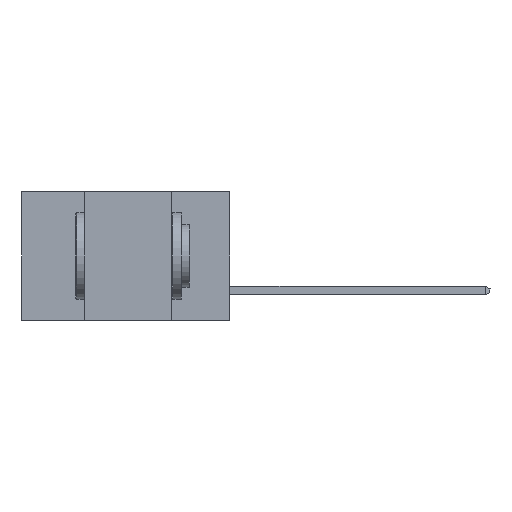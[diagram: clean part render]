
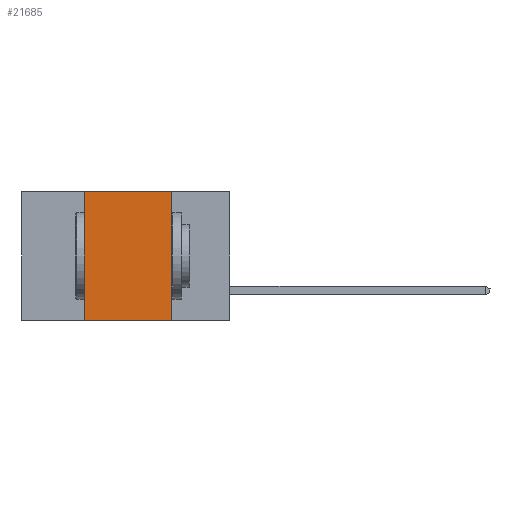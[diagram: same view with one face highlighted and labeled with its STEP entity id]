
A CAD part, left-side view. The second image highlights one B-rep face of the part: STEP entity #21685.
In plain terms, the highlighted planar face has unit normal (-1, 0, 0).
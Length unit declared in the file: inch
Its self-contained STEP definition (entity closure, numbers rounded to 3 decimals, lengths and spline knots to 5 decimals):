
#300 = PLANE ( 'NONE',  #4115 ) ;
#487 = ORIENTED_EDGE ( 'NONE', *, *, #19760, .T. ) ;
#1182 = CARTESIAN_POINT ( 'NONE',  ( 0., 0.42, -0.37 ) ) ;
#2462 = LINE ( 'NONE', #9698, #23438 ) ;
#3084 = DIRECTION ( 'NONE',  ( 0., 0., -1. ) ) ;
#3310 = EDGE_CURVE ( 'NONE', #15651, #19682, #10337, .T. ) ;
#3701 = CARTESIAN_POINT ( 'NONE',  ( 0., 0.6, 0. ) ) ;
#3824 = DIRECTION ( 'NONE',  ( 0., -1., 0. ) ) ;
#4115 = AXIS2_PLACEMENT_3D ( 'NONE', #7672, #5869, #23579 ) ;
#5869 = DIRECTION ( 'NONE',  ( 1., 0., 0. ) ) ;
#6494 = VERTEX_POINT ( 'NONE', #7922 ) ;
#7672 = CARTESIAN_POINT ( 'NONE',  ( 0., 0.6, 0. ) ) ;
#7922 = CARTESIAN_POINT ( 'NONE',  ( 0., 0.17, -0.37 ) ) ;
#9698 = CARTESIAN_POINT ( 'NONE',  ( 0., 0.6, -0.37 ) ) ;
#10337 = LINE ( 'NONE', #1182, #10349 ) ;
#10349 = VECTOR ( 'NONE', #19405, 39.37008 ) ;
#10503 = CARTESIAN_POINT ( 'NONE',  ( 0., 0.42, -0.37 ) ) ;
#11287 = FACE_OUTER_BOUND ( 'NONE', #11993, .T. ) ;
#11993 = EDGE_LOOP ( 'NONE', ( #12324, #22011, #21460, #487 ) ) ;
#12139 = VECTOR ( 'NONE', #3084, 39.37008 ) ;
#12266 = LINE ( 'NONE', #19635, #12139 ) ;
#12324 = ORIENTED_EDGE ( 'NONE', *, *, #15439, .F. ) ;
#12665 = CARTESIAN_POINT ( 'NONE',  ( 0., 0.17, 0. ) ) ;
#13090 = DIRECTION ( 'NONE',  ( 0., -1., 0. ) ) ;
#15252 = CARTESIAN_POINT ( 'NONE',  ( 0., 0.42, 0. ) ) ;
#15439 = EDGE_CURVE ( 'NONE', #18734, #6494, #12266, .T. ) ;
#15651 = VERTEX_POINT ( 'NONE', #10503 ) ;
#16233 = LINE ( 'NONE', #3701, #19960 ) ;
#18734 = VERTEX_POINT ( 'NONE', #12665 ) ;
#19405 = DIRECTION ( 'NONE',  ( 0., 0., 1. ) ) ;
#19611 = EDGE_CURVE ( 'NONE', #19682, #18734, #16233, .T. ) ;
#19635 = CARTESIAN_POINT ( 'NONE',  ( 0., 0.17, -0.37 ) ) ;
#19682 = VERTEX_POINT ( 'NONE', #15252 ) ;
#19760 = EDGE_CURVE ( 'NONE', #15651, #6494, #2462, .T. ) ;
#19960 = VECTOR ( 'NONE', #3824, 39.37008 ) ;
#21460 = ORIENTED_EDGE ( 'NONE', *, *, #3310, .F. ) ;
#21685 = ADVANCED_FACE ( 'NONE', ( #11287 ), #300, .F. ) ;
#22011 = ORIENTED_EDGE ( 'NONE', *, *, #19611, .F. ) ;
#23438 = VECTOR ( 'NONE', #13090, 39.37008 ) ;
#23579 = DIRECTION ( 'NONE',  ( 0., 0., -1. ) ) ;
